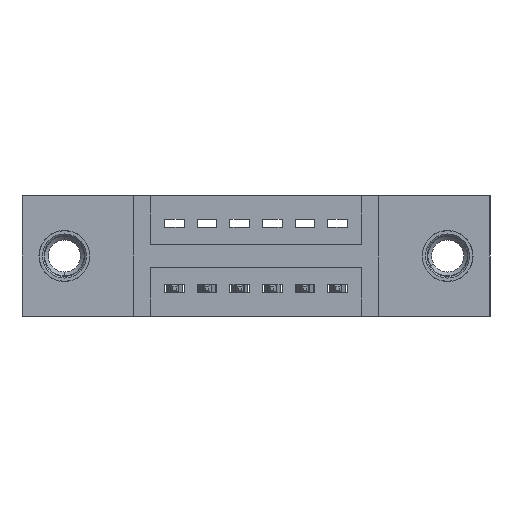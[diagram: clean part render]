
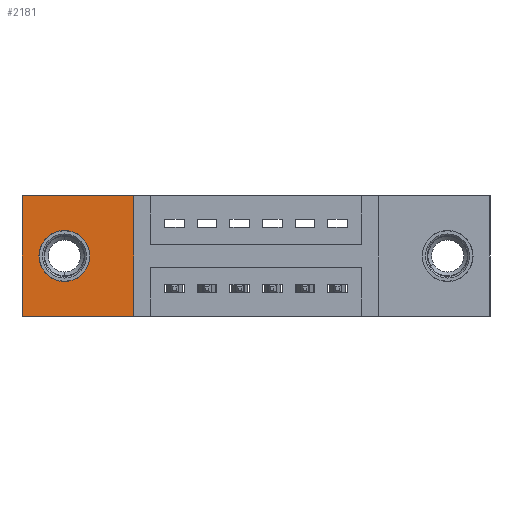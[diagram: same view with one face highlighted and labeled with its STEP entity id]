
A CAD part, front view. The second image highlights one B-rep face of the part: STEP entity #2181.
In plain terms, the highlighted planar face has unit normal (0, -1, 0).
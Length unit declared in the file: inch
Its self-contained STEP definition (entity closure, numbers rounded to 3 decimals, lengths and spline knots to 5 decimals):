
#500 = CARTESIAN_POINT ( 'NONE',  ( 0., 0.11, 0. ) ) ;
#559 = CARTESIAN_POINT ( 'NONE',  ( 0.3425, 0.11, -0.37 ) ) ;
#694 = CIRCLE ( 'NONE', #890, 0.078 ) ;
#749 = CARTESIAN_POINT ( 'NONE',  ( 0., 0.11, -0.37 ) ) ;
#833 = CARTESIAN_POINT ( 'NONE',  ( 0.13, 0.11, -0.185 ) ) ;
#872 = DIRECTION ( 'NONE',  ( 0., -1., 0. ) ) ;
#875 = DIRECTION ( 'NONE',  ( 0., 0., -1. ) ) ;
#890 = AXIS2_PLACEMENT_3D ( 'NONE', #833, #872, #875 ) ;
#1108 = CARTESIAN_POINT ( 'NONE',  ( 0.13, 0.11, -0.263 ) ) ;
#1315 = EDGE_LOOP ( 'NONE', ( #2980, #9302, #3508, #10205 ) ) ;
#1834 = EDGE_LOOP ( 'NONE', ( #7421, #6562 ) ) ;
#1879 = VERTEX_POINT ( 'NONE', #2419 ) ;
#1964 = CARTESIAN_POINT ( 'NONE',  ( 0., 0.11, 0. ) ) ;
#2181 = ADVANCED_FACE ( 'NONE', ( #2208, #9922 ), #4464, .T. ) ;
#2208 = FACE_BOUND ( 'NONE', #1834, .T. ) ;
#2419 = CARTESIAN_POINT ( 'NONE',  ( 0., 0.11, -0.37 ) ) ;
#2573 = VERTEX_POINT ( 'NONE', #7531 ) ;
#2669 = VECTOR ( 'NONE', #4644, 39.37008 ) ;
#2726 = DIRECTION ( 'NONE',  ( 1., 0., 0. ) ) ;
#2980 = ORIENTED_EDGE ( 'NONE', *, *, #9046, .T. ) ;
#3372 = VECTOR ( 'NONE', #2726, 39.37008 ) ;
#3375 = DIRECTION ( 'NONE',  ( 0., 0., -1. ) ) ;
#3508 = ORIENTED_EDGE ( 'NONE', *, *, #6117, .T. ) ;
#3628 = LINE ( 'NONE', #749, #3372 ) ;
#4028 = EDGE_CURVE ( 'NONE', #10115, #4825, #4157, .T. ) ;
#4119 = CARTESIAN_POINT ( 'NONE',  ( 0.3425, 0.11, 0. ) ) ;
#4157 = CIRCLE ( 'NONE', #6931, 0.078 ) ;
#4424 = CARTESIAN_POINT ( 'NONE',  ( 0., 0.11, -0.37 ) ) ;
#4464 = PLANE ( 'NONE',  #7003 ) ;
#4470 = CARTESIAN_POINT ( 'NONE',  ( 0.13, 0.11, -0.107 ) ) ;
#4644 = DIRECTION ( 'NONE',  ( -1., 0., 0. ) ) ;
#4652 = LINE ( 'NONE', #9297, #2669 ) ;
#4825 = VERTEX_POINT ( 'NONE', #1108 ) ;
#5008 = DIRECTION ( 'NONE',  ( 0., 0., 1. ) ) ;
#5273 = EDGE_CURVE ( 'NONE', #4825, #10115, #694, .T. ) ;
#5550 = VERTEX_POINT ( 'NONE', #559 ) ;
#5851 = DIRECTION ( 'NONE',  ( 0., 0., -1. ) ) ;
#5864 = DIRECTION ( 'NONE',  ( 0., -1., 0. ) ) ;
#5866 = CARTESIAN_POINT ( 'NONE',  ( 0.13, 0.11, -0.185 ) ) ;
#6117 = EDGE_CURVE ( 'NONE', #5550, #2573, #8597, .T. ) ;
#6171 = DIRECTION ( 'NONE',  ( 0., 0., -1. ) ) ;
#6562 = ORIENTED_EDGE ( 'NONE', *, *, #5273, .F. ) ;
#6768 = DIRECTION ( 'NONE',  ( 0., -1., 0. ) ) ;
#6931 = AXIS2_PLACEMENT_3D ( 'NONE', #5866, #5864, #5851 ) ;
#6945 = EDGE_CURVE ( 'NONE', #1879, #5550, #3628, .T. ) ;
#7003 = AXIS2_PLACEMENT_3D ( 'NONE', #4424, #6768, #3375 ) ;
#7421 = ORIENTED_EDGE ( 'NONE', *, *, #4028, .F. ) ;
#7531 = CARTESIAN_POINT ( 'NONE',  ( 0.3425, 0.11, 0. ) ) ;
#8590 = EDGE_CURVE ( 'NONE', #2573, #9364, #4652, .T. ) ;
#8597 = LINE ( 'NONE', #4119, #9873 ) ;
#8774 = LINE ( 'NONE', #1964, #10275 ) ;
#9046 = EDGE_CURVE ( 'NONE', #9364, #1879, #8774, .T. ) ;
#9297 = CARTESIAN_POINT ( 'NONE',  ( 0., 0.11, 0. ) ) ;
#9302 = ORIENTED_EDGE ( 'NONE', *, *, #6945, .T. ) ;
#9364 = VERTEX_POINT ( 'NONE', #500 ) ;
#9873 = VECTOR ( 'NONE', #5008, 39.37008 ) ;
#9922 = FACE_OUTER_BOUND ( 'NONE', #1315, .T. ) ;
#10115 = VERTEX_POINT ( 'NONE', #4470 ) ;
#10205 = ORIENTED_EDGE ( 'NONE', *, *, #8590, .T. ) ;
#10275 = VECTOR ( 'NONE', #6171, 39.37008 ) ;
